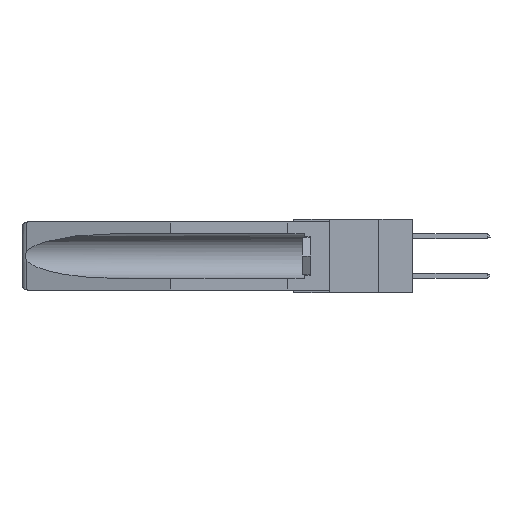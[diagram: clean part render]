
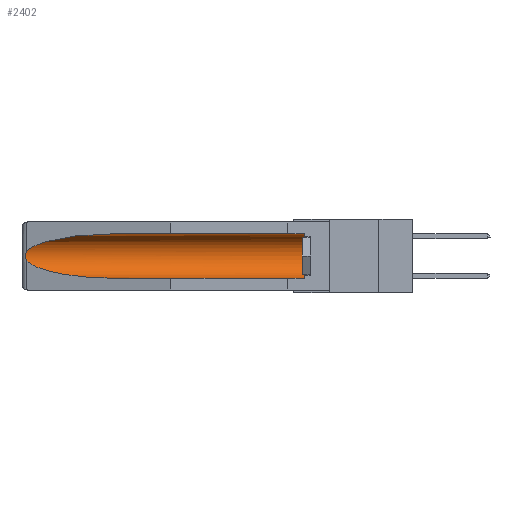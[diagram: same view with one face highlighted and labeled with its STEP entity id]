
A CAD part, left-side view. The second image highlights one B-rep face of the part: STEP entity #2402.
In plain terms, the highlighted cylindrical face has radius 2.857 mm (diameter 5.715 mm), a partial arc.
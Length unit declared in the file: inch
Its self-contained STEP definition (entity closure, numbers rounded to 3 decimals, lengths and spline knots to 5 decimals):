
#153 = EDGE_CURVE ( 'NONE', #18303, #5354, #4914, .T. ) ;
#282 = B_SPLINE_CURVE_WITH_KNOTS ( 'NONE', 3,
 ( #14017, #2456, #19568, #15598, #4465, #17906, #8105, #10004, #11921, #530 ),
 .UNSPECIFIED., .F., .F.,
 ( 4, 2, 2, 2, 4 ),
 ( 0., 0.00029, 0.00058, 0.00087, 0.00117 ),
 .UNSPECIFIED. ) ;
#351 = ORIENTED_EDGE ( 'NONE', *, *, #7409, .T. ) ;
#530 = CARTESIAN_POINT ( 'NONE',  ( 0.26537, 1.52718, -0.19328 ) ) ;
#1198 = CARTESIAN_POINT ( 'NONE',  ( 0.155, 1.07973, -0.284 ) ) ;
#1499 = CARTESIAN_POINT ( 'NONE',  ( 0.155, -0.30754, -0.059 ) ) ;
#1627 = CARTESIAN_POINT ( 'NONE',  ( 0.26537, 1.52718, -0.14972 ) ) ;
#1748 = EDGE_CURVE ( 'NONE', #5354, #7813, #18688, .T. ) ;
#2402 = ADVANCED_FACE ( 'NONE', ( #8763 ), #18080, .F. ) ;
#2417 = CARTESIAN_POINT ( 'NONE',  ( 0.26537, 1.52718, -0.14972 ) ) ;
#2456 = CARTESIAN_POINT ( 'NONE',  ( 0.26597, 1.52961, -0.15275 ) ) ;
#2865 = CARTESIAN_POINT ( 'NONE',  ( 0.155, 1.07973, -0.284 ) ) ;
#3308 = DIRECTION ( 'NONE',  ( 0., -1., 0. ) ) ;
#3362 = LINE ( 'NONE', #13728, #12957 ) ;
#3762 = CARTESIAN_POINT ( 'NONE',  ( 0.155, -0.30754, -0.1715 ) ) ;
#4465 = CARTESIAN_POINT ( 'NONE',  ( 0.2675, 1.53308, -0.16763 ) ) ;
#4807 = ORIENTED_EDGE ( 'NONE', *, *, #1748, .T. ) ;
#4914 = CIRCLE ( 'NONE', #8138, 0.1125 ) ;
#5354 = VERTEX_POINT ( 'NONE', #6908 ) ;
#6061 = ORIENTED_EDGE ( 'NONE', *, *, #8507, .T. ) ;
#6606 = EDGE_CURVE ( 'NONE', #18303, #12738, #3362, .T. ) ;
#6908 = CARTESIAN_POINT ( 'NONE',  ( 0.155, 0.126, -0.059 ) ) ;
#7155 = DIRECTION ( 'NONE',  ( 0., 0., 1. ) ) ;
#7409 = EDGE_CURVE ( 'NONE', #12870, #12738, #15770, .T. ) ;
#7813 = VERTEX_POINT ( 'NONE', #24700 ) ;
#8105 = CARTESIAN_POINT ( 'NONE',  ( 0.2673, 1.53269, -0.17917 ) ) ;
#8138 = AXIS2_PLACEMENT_3D ( 'NONE', #14788, #3308, #7155 ) ;
#8507 = EDGE_CURVE ( 'NONE', #7813, #11751, #13155, .T. ) ;
#8763 = FACE_OUTER_BOUND ( 'NONE', #12270, .T. ) ;
#10004 = CARTESIAN_POINT ( 'NONE',  ( 0.26655, 1.53094, -0.18657 ) ) ;
#10417 = AXIS2_PLACEMENT_3D ( 'NONE', #3762, #19139, #15252 ) ;
#10506 = CARTESIAN_POINT ( 'NONE',  ( 0.26537, 1.52718, -0.19328 ) ) ;
#11751 = VERTEX_POINT ( 'NONE', #2417 ) ;
#11921 = CARTESIAN_POINT ( 'NONE',  ( 0.26597, 1.5296, -0.19026 ) ) ;
#12270 = EDGE_LOOP ( 'NONE', ( #6061, #12593, #351, #24470, #14302, #4807 ) ) ;
#12340 = CARTESIAN_POINT ( 'NONE',  ( 0.25451, 1.48313, -0.24835 ) ) ;
#12424 = DIRECTION ( 'NONE',  ( 0., 1., 0. ) ) ;
#12593 = ORIENTED_EDGE ( 'NONE', *, *, #22158, .T. ) ;
#12738 = VERTEX_POINT ( 'NONE', #1198 ) ;
#12870 = VERTEX_POINT ( 'NONE', #18809 ) ;
#12957 = VECTOR ( 'NONE', #17698, 39.37008 ) ;
#13155 =( BOUNDED_CURVE ( )  B_SPLINE_CURVE ( 3, ( #22550, #18611, #24398, #1627 ),
 .UNSPECIFIED., .F., .F. ) 
 B_SPLINE_CURVE_WITH_KNOTS ( ( 4, 4 ),
 ( 4.71239, 6.08839 ),
 .UNSPECIFIED. ) 
 CURVE ( )  GEOMETRIC_REPRESENTATION_ITEM ( )  RATIONAL_B_SPLINE_CURVE ( ( 1., 0.848, 0.848, 1. ) ) 
 REPRESENTATION_ITEM ( '' )  );
#13728 = CARTESIAN_POINT ( 'NONE',  ( 0.155, -0.30754, -0.284 ) ) ;
#14017 = CARTESIAN_POINT ( 'NONE',  ( 0.26537, 1.52718, -0.14972 ) ) ;
#14302 = ORIENTED_EDGE ( 'NONE', *, *, #153, .T. ) ;
#14788 = CARTESIAN_POINT ( 'NONE',  ( 0.155, 0.126, -0.1715 ) ) ;
#15252 = DIRECTION ( 'NONE',  ( 0., 0., 1. ) ) ;
#15598 = CARTESIAN_POINT ( 'NONE',  ( 0.2673, 1.5327, -0.16383 ) ) ;
#15770 =( BOUNDED_CURVE ( )  B_SPLINE_CURVE ( 3, ( #10506, #12340, #20144, #2865 ),
 .UNSPECIFIED., .F., .F. ) 
 B_SPLINE_CURVE_WITH_KNOTS ( ( 4, 4 ),
 ( 0.1948, 1.5708 ),
 .UNSPECIFIED. ) 
 CURVE ( )  GEOMETRIC_REPRESENTATION_ITEM ( )  RATIONAL_B_SPLINE_CURVE ( ( 1., 0.848, 0.848, 1. ) ) 
 REPRESENTATION_ITEM ( '' )  );
#17698 = DIRECTION ( 'NONE',  ( 0., 1., 0. ) ) ;
#17906 = CARTESIAN_POINT ( 'NONE',  ( 0.2675, 1.53308, -0.17534 ) ) ;
#18080 = CYLINDRICAL_SURFACE ( 'NONE', #10417, 0.1125 ) ;
#18303 = VERTEX_POINT ( 'NONE', #20452 ) ;
#18413 = VECTOR ( 'NONE', #12424, 39.37008 ) ;
#18611 = CARTESIAN_POINT ( 'NONE',  ( 0.21114, 1.30732, -0.059 ) ) ;
#18688 = LINE ( 'NONE', #1499, #18413 ) ;
#18809 = CARTESIAN_POINT ( 'NONE',  ( 0.26537, 1.52718, -0.19328 ) ) ;
#19139 = DIRECTION ( 'NONE',  ( 0., 1., 0. ) ) ;
#19568 = CARTESIAN_POINT ( 'NONE',  ( 0.26654, 1.53092, -0.15636 ) ) ;
#20144 = CARTESIAN_POINT ( 'NONE',  ( 0.21114, 1.30732, -0.284 ) ) ;
#20452 = CARTESIAN_POINT ( 'NONE',  ( 0.155, 0.126, -0.284 ) ) ;
#22158 = EDGE_CURVE ( 'NONE', #11751, #12870, #282, .T. ) ;
#22550 = CARTESIAN_POINT ( 'NONE',  ( 0.155, 1.07973, -0.059 ) ) ;
#24398 = CARTESIAN_POINT ( 'NONE',  ( 0.25451, 1.48313, -0.09465 ) ) ;
#24470 = ORIENTED_EDGE ( 'NONE', *, *, #6606, .F. ) ;
#24700 = CARTESIAN_POINT ( 'NONE',  ( 0.155, 1.07973, -0.059 ) ) ;
